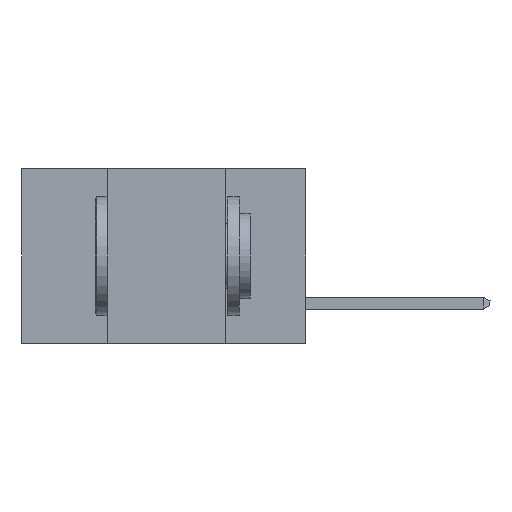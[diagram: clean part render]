
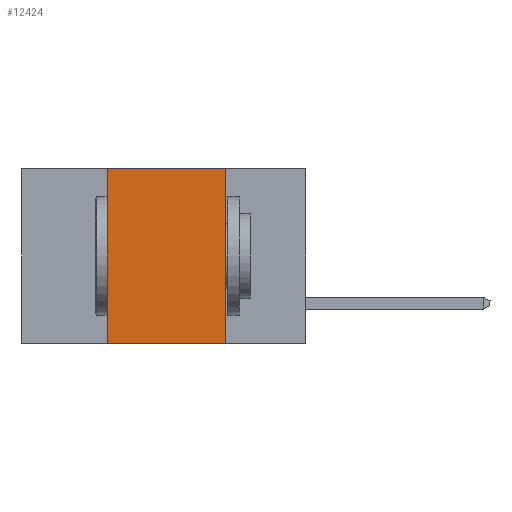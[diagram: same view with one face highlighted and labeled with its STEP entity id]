
A CAD part, left-side view. The second image highlights one B-rep face of the part: STEP entity #12424.
In plain terms, the highlighted planar face has unit normal (-1, 0, 0).
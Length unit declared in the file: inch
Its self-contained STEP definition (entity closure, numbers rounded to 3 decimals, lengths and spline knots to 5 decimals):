
#384 = EDGE_CURVE ( 'NONE', #8041, #18725, #6056, .T. ) ;
#893 = DIRECTION ( 'NONE',  ( 0., 0., -1. ) ) ;
#1183 = VECTOR ( 'NONE', #893, 39.37008 ) ;
#1649 = EDGE_CURVE ( 'NONE', #8041, #12594, #18272, .T. ) ;
#3158 = CARTESIAN_POINT ( 'NONE',  ( 0., 0.6, 0. ) ) ;
#3612 = ORIENTED_EDGE ( 'NONE', *, *, #384, .T. ) ;
#4687 = PLANE ( 'NONE',  #15709 ) ;
#5092 = CARTESIAN_POINT ( 'NONE',  ( 0., 0.17, 0. ) ) ;
#5133 = CARTESIAN_POINT ( 'NONE',  ( 0., 0.42, -0.37 ) ) ;
#5171 = LINE ( 'NONE', #18277, #1183 ) ;
#5376 = LINE ( 'NONE', #18489, #17567 ) ;
#5837 = DIRECTION ( 'NONE',  ( 0., 0., -1. ) ) ;
#6056 = LINE ( 'NONE', #8981, #17527 ) ;
#6920 = EDGE_CURVE ( 'NONE', #12594, #15157, #5376, .T. ) ;
#8003 = EDGE_LOOP ( 'NONE', ( #15174, #15280, #13329, #3612 ) ) ;
#8041 = VERTEX_POINT ( 'NONE', #5133 ) ;
#8210 = CARTESIAN_POINT ( 'NONE',  ( 0., 0.42, -0.37 ) ) ;
#8981 = CARTESIAN_POINT ( 'NONE',  ( 0., 0.6, -0.37 ) ) ;
#10012 = CARTESIAN_POINT ( 'NONE',  ( 0., 0.17, -0.37 ) ) ;
#10202 = FACE_OUTER_BOUND ( 'NONE', #8003, .T. ) ;
#11367 = DIRECTION ( 'NONE',  ( 0., -1., 0. ) ) ;
#12144 = EDGE_CURVE ( 'NONE', #15157, #18725, #5171, .T. ) ;
#12424 = ADVANCED_FACE ( 'NONE', ( #10202 ), #4687, .F. ) ;
#12594 = VERTEX_POINT ( 'NONE', #14165 ) ;
#13329 = ORIENTED_EDGE ( 'NONE', *, *, #1649, .F. ) ;
#13998 = DIRECTION ( 'NONE',  ( 0., 0., 1. ) ) ;
#14165 = CARTESIAN_POINT ( 'NONE',  ( 0., 0.42, 0. ) ) ;
#15157 = VERTEX_POINT ( 'NONE', #5092 ) ;
#15174 = ORIENTED_EDGE ( 'NONE', *, *, #12144, .F. ) ;
#15280 = ORIENTED_EDGE ( 'NONE', *, *, #6920, .F. ) ;
#15709 = AXIS2_PLACEMENT_3D ( 'NONE', #3158, #16270, #5837 ) ;
#15812 = VECTOR ( 'NONE', #13998, 39.37008 ) ;
#16270 = DIRECTION ( 'NONE',  ( 1., 0., 0. ) ) ;
#17527 = VECTOR ( 'NONE', #17635, 39.37008 ) ;
#17567 = VECTOR ( 'NONE', #11367, 39.37008 ) ;
#17635 = DIRECTION ( 'NONE',  ( 0., -1., 0. ) ) ;
#18272 = LINE ( 'NONE', #8210, #15812 ) ;
#18277 = CARTESIAN_POINT ( 'NONE',  ( 0., 0.17, -0.37 ) ) ;
#18489 = CARTESIAN_POINT ( 'NONE',  ( 0., 0.6, 0. ) ) ;
#18725 = VERTEX_POINT ( 'NONE', #10012 ) ;
